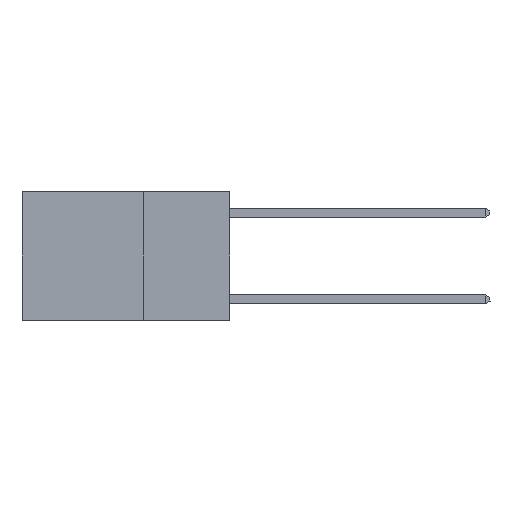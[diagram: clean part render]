
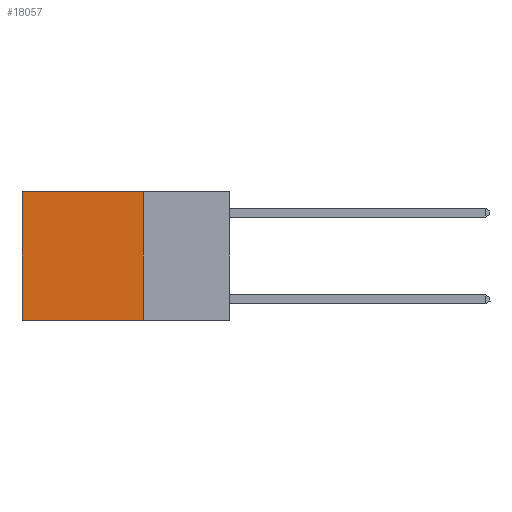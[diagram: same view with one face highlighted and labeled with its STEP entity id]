
A CAD part, left-side view. The second image highlights one B-rep face of the part: STEP entity #18057.
In plain terms, the highlighted planar face has unit normal (-1, 0, 0).
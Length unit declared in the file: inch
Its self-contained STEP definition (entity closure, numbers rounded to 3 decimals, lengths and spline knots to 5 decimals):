
#38 = VECTOR ( 'NONE', #14461, 39.37008 ) ;
#661 = ORIENTED_EDGE ( 'NONE', *, *, #18060, .F. ) ;
#2136 = FACE_OUTER_BOUND ( 'NONE', #8086, .T. ) ;
#2256 = ORIENTED_EDGE ( 'NONE', *, *, #7244, .F. ) ;
#3118 = CARTESIAN_POINT ( 'NONE',  ( 0.2625, 0.25, -0.37 ) ) ;
#3340 = ORIENTED_EDGE ( 'NONE', *, *, #4210, .T. ) ;
#4210 = EDGE_CURVE ( 'NONE', #11821, #13777, #13998, .T. ) ;
#5208 = DIRECTION ( 'NONE',  ( 1., 0., 0. ) ) ;
#6608 = LINE ( 'NONE', #14469, #9854 ) ;
#7244 = EDGE_CURVE ( 'NONE', #14190, #13777, #8659, .T. ) ;
#8086 = EDGE_LOOP ( 'NONE', ( #3340, #2256, #661, #12338 ) ) ;
#8659 = LINE ( 'NONE', #3118, #10407 ) ;
#8733 = DIRECTION ( 'NONE',  ( 0., 1., 0. ) ) ;
#8853 = VECTOR ( 'NONE', #10930, 39.37008 ) ;
#9382 = CARTESIAN_POINT ( 'NONE',  ( 0.2625, 0.25, 0. ) ) ;
#9854 = VECTOR ( 'NONE', #14364, 39.37008 ) ;
#10275 = EDGE_CURVE ( 'NONE', #16247, #11821, #6608, .T. ) ;
#10407 = VECTOR ( 'NONE', #8733, 39.37008 ) ;
#10845 = LINE ( 'NONE', #17973, #8853 ) ;
#10930 = DIRECTION ( 'NONE',  ( 0., 0., -1. ) ) ;
#11599 = CARTESIAN_POINT ( 'NONE',  ( 0.2625, 0.6, 0. ) ) ;
#11821 = VERTEX_POINT ( 'NONE', #17686 ) ;
#12338 = ORIENTED_EDGE ( 'NONE', *, *, #10275, .T. ) ;
#13777 = VERTEX_POINT ( 'NONE', #16322 ) ;
#13998 = LINE ( 'NONE', #11599, #38 ) ;
#14190 = VERTEX_POINT ( 'NONE', #17346 ) ;
#14364 = DIRECTION ( 'NONE',  ( 0., 1., 0. ) ) ;
#14461 = DIRECTION ( 'NONE',  ( 0., 0., -1. ) ) ;
#14469 = CARTESIAN_POINT ( 'NONE',  ( 0.2625, 0.25, 0. ) ) ;
#14687 = CARTESIAN_POINT ( 'NONE',  ( 0.2625, 0.25, 0. ) ) ;
#15118 = DIRECTION ( 'NONE',  ( 0., 0., -1. ) ) ;
#16247 = VERTEX_POINT ( 'NONE', #14687 ) ;
#16322 = CARTESIAN_POINT ( 'NONE',  ( 0.2625, 0.6, -0.37 ) ) ;
#16609 = PLANE ( 'NONE',  #18023 ) ;
#17346 = CARTESIAN_POINT ( 'NONE',  ( 0.2625, 0.25, -0.37 ) ) ;
#17686 = CARTESIAN_POINT ( 'NONE',  ( 0.2625, 0.6, 0. ) ) ;
#17973 = CARTESIAN_POINT ( 'NONE',  ( 0.2625, 0.25, 0. ) ) ;
#18023 = AXIS2_PLACEMENT_3D ( 'NONE', #9382, #5208, #15118 ) ;
#18057 = ADVANCED_FACE ( 'NONE', ( #2136 ), #16609, .F. ) ;
#18060 = EDGE_CURVE ( 'NONE', #16247, #14190, #10845, .T. ) ;
